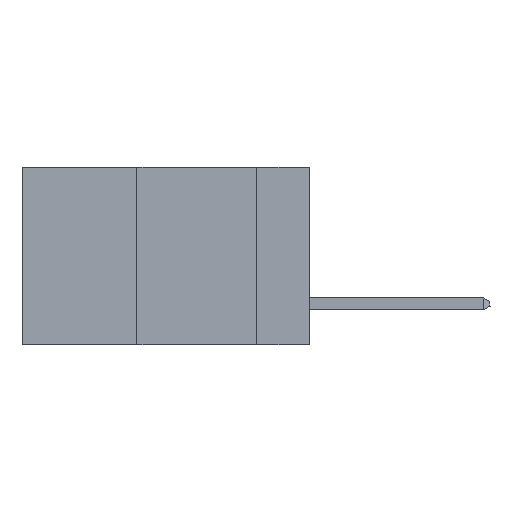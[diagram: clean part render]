
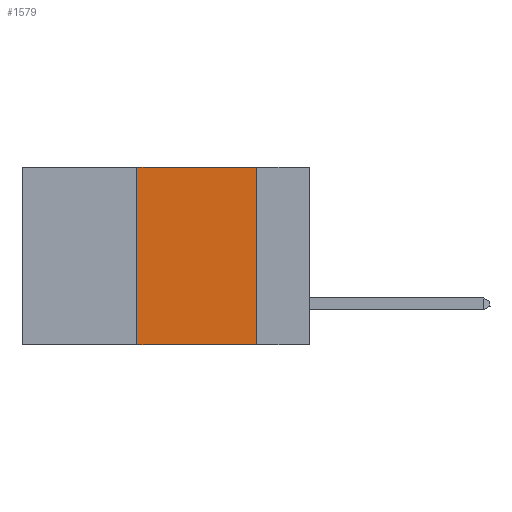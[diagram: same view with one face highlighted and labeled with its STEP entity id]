
A CAD part, left-side view. The second image highlights one B-rep face of the part: STEP entity #1579.
In plain terms, the highlighted planar face has unit normal (-1, 0, 0).
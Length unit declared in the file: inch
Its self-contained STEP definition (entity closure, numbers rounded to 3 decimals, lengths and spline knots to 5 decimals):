
#1230 = DIRECTION ( 'NONE',  ( 0., 0., -1. ) ) ;
#1426 = DIRECTION ( 'NONE',  ( 1., 0., 0. ) ) ;
#1579 = ADVANCED_FACE ( 'NONE', ( #21778 ), #15682, .F. ) ;
#2980 = LINE ( 'NONE', #11215, #4447 ) ;
#3166 = DIRECTION ( 'NONE',  ( 0., 0., -1. ) ) ;
#4150 = ORIENTED_EDGE ( 'NONE', *, *, #19089, .T. ) ;
#4266 = DIRECTION ( 'NONE',  ( 0., -1., 0. ) ) ;
#4447 = VECTOR ( 'NONE', #1230, 39.37008 ) ;
#6099 = CARTESIAN_POINT ( 'NONE',  ( 0., 0.36, 0. ) ) ;
#7451 = VECTOR ( 'NONE', #4266, 39.37008 ) ;
#7682 = VERTEX_POINT ( 'NONE', #11865 ) ;
#7820 = VERTEX_POINT ( 'NONE', #10499 ) ;
#8789 = LINE ( 'NONE', #6099, #19028 ) ;
#9121 = CARTESIAN_POINT ( 'NONE',  ( 0., 0.11, 0. ) ) ;
#9709 = VERTEX_POINT ( 'NONE', #9121 ) ;
#10499 = CARTESIAN_POINT ( 'NONE',  ( 0., 0.36, -0.37 ) ) ;
#10550 = ORIENTED_EDGE ( 'NONE', *, *, #13174, .F. ) ;
#10651 = EDGE_CURVE ( 'NONE', #13070, #9709, #14759, .T. ) ;
#10852 = DIRECTION ( 'NONE',  ( 0., -1., 0. ) ) ;
#11215 = CARTESIAN_POINT ( 'NONE',  ( 0., 0.11, 0. ) ) ;
#11865 = CARTESIAN_POINT ( 'NONE',  ( 0., 0.11, -0.37 ) ) ;
#13070 = VERTEX_POINT ( 'NONE', #26047 ) ;
#13174 = EDGE_CURVE ( 'NONE', #7820, #13070, #8789, .T. ) ;
#14759 = LINE ( 'NONE', #18946, #7451 ) ;
#15682 = PLANE ( 'NONE',  #22735 ) ;
#16658 = EDGE_CURVE ( 'NONE', #9709, #7682, #2980, .T. ) ;
#18946 = CARTESIAN_POINT ( 'NONE',  ( 0., 0.6, 0. ) ) ;
#19028 = VECTOR ( 'NONE', #22550, 39.37008 ) ;
#19089 = EDGE_CURVE ( 'NONE', #7820, #7682, #21093, .T. ) ;
#21093 = LINE ( 'NONE', #23237, #23470 ) ;
#21778 = FACE_OUTER_BOUND ( 'NONE', #22957, .T. ) ;
#22550 = DIRECTION ( 'NONE',  ( 0., 0., 1. ) ) ;
#22735 = AXIS2_PLACEMENT_3D ( 'NONE', #23793, #1426, #3166 ) ;
#22957 = EDGE_LOOP ( 'NONE', ( #25763, #26510, #10550, #4150 ) ) ;
#23237 = CARTESIAN_POINT ( 'NONE',  ( 0., 0.6, -0.37 ) ) ;
#23470 = VECTOR ( 'NONE', #10852, 39.37008 ) ;
#23793 = CARTESIAN_POINT ( 'NONE',  ( 0., 0.6, 0. ) ) ;
#25763 = ORIENTED_EDGE ( 'NONE', *, *, #16658, .F. ) ;
#26047 = CARTESIAN_POINT ( 'NONE',  ( 0., 0.36, 0. ) ) ;
#26510 = ORIENTED_EDGE ( 'NONE', *, *, #10651, .F. ) ;
